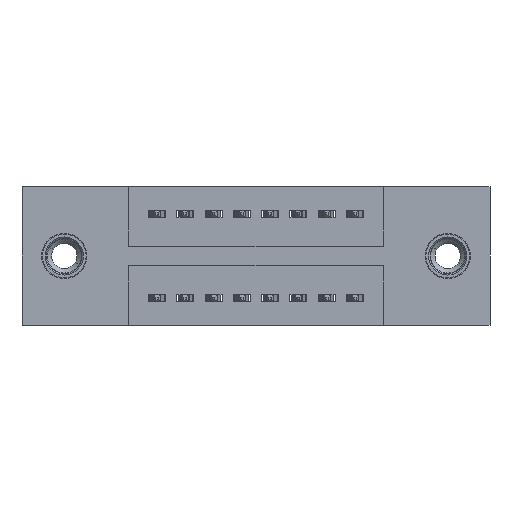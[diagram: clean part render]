
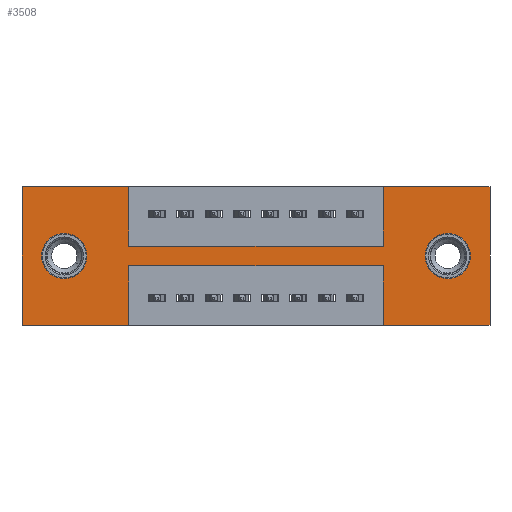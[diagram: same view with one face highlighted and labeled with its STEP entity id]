
A CAD part, front view. The second image highlights one B-rep face of the part: STEP entity #3508.
In plain terms, the highlighted planar face has unit normal (0, -1, 0).
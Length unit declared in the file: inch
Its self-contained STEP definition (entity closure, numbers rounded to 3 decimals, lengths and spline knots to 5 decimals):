
#257 = VERTEX_POINT ( 'NONE', #9334 ) ;
#258 = DIRECTION ( 'NONE',  ( 0., 1., 0. ) ) ;
#291 = CARTESIAN_POINT ( 'NONE',  ( 0.3775, 0., -0.28 ) ) ;
#521 = EDGE_CURVE ( 'NONE', #3540, #8473, #681, .T. ) ;
#585 = CARTESIAN_POINT ( 'NONE',  ( 1.655, 0., 0. ) ) ;
#623 = CARTESIAN_POINT ( 'NONE',  ( 1.655, 0., 0. ) ) ;
#681 = LINE ( 'NONE', #2844, #2631 ) ;
#764 = AXIS2_PLACEMENT_3D ( 'NONE', #10025, #2555, #10059 ) ;
#872 = EDGE_LOOP ( 'NONE', ( #3170, #6755 ) ) ;
#934 = DIRECTION ( 'NONE',  ( -1., 0., 0. ) ) ;
#1196 = ORIENTED_EDGE ( 'NONE', *, *, #9665, .F. ) ;
#1228 = CARTESIAN_POINT ( 'NONE',  ( 0., 0., -0.49 ) ) ;
#1275 = LINE ( 'NONE', #1695, #3624 ) ;
#1340 = VECTOR ( 'NONE', #8317, 39.37008 ) ;
#1508 = VERTEX_POINT ( 'NONE', #7188 ) ;
#1526 = LINE ( 'NONE', #4250, #10143 ) ;
#1599 = VERTEX_POINT ( 'NONE', #10474 ) ;
#1629 = VERTEX_POINT ( 'NONE', #10762 ) ;
#1646 = EDGE_CURVE ( 'NONE', #1508, #257, #7948, .T. ) ;
#1695 = CARTESIAN_POINT ( 'NONE',  ( 0., 0., -0.49 ) ) ;
#1846 = VECTOR ( 'NONE', #7177, 39.37008 ) ;
#1883 = DIRECTION ( 'NONE',  ( 0., 1., 0. ) ) ;
#2124 = CARTESIAN_POINT ( 'NONE',  ( 0., 0., 0. ) ) ;
#2167 = DIRECTION ( 'NONE',  ( 0., 0., -1. ) ) ;
#2207 = EDGE_CURVE ( 'NONE', #7384, #5151, #1275, .T. ) ;
#2238 = ORIENTED_EDGE ( 'NONE', *, *, #1646, .T. ) ;
#2365 = DIRECTION ( 'NONE',  ( 0., 0., -1. ) ) ;
#2447 = CIRCLE ( 'NONE', #764, 0.08 ) ;
#2555 = DIRECTION ( 'NONE',  ( 0., 1., 0. ) ) ;
#2631 = VECTOR ( 'NONE', #10314, 39.37008 ) ;
#2638 = CARTESIAN_POINT ( 'NONE',  ( 1.5055, 0., -0.245 ) ) ;
#2647 = ORIENTED_EDGE ( 'NONE', *, *, #8087, .F. ) ;
#2670 = ORIENTED_EDGE ( 'NONE', *, *, #3336, .F. ) ;
#2773 = EDGE_CURVE ( 'NONE', #7735, #1629, #1526, .T. ) ;
#2844 = CARTESIAN_POINT ( 'NONE',  ( 0., 0., -0.49 ) ) ;
#3000 = VERTEX_POINT ( 'NONE', #10274 ) ;
#3110 = AXIS2_PLACEMENT_3D ( 'NONE', #6658, #6697, #7510 ) ;
#3155 = CIRCLE ( 'NONE', #3383, 0.08 ) ;
#3166 = EDGE_LOOP ( 'NONE', ( #4093, #2238 ) ) ;
#3170 = ORIENTED_EDGE ( 'NONE', *, *, #5149, .T. ) ;
#3336 = EDGE_CURVE ( 'NONE', #1599, #9277, #3474, .T. ) ;
#3383 = AXIS2_PLACEMENT_3D ( 'NONE', #8575, #1883, #10221 ) ;
#3471 = VECTOR ( 'NONE', #2167, 39.37008 ) ;
#3474 = LINE ( 'NONE', #6778, #10266 ) ;
#3477 = ORIENTED_EDGE ( 'NONE', *, *, #2773, .F. ) ;
#3508 = ADVANCED_FACE ( 'NONE', ( #10252, #8301, #4794 ), #3770, .T. ) ;
#3540 = VERTEX_POINT ( 'NONE', #10417 ) ;
#3578 = CIRCLE ( 'NONE', #3110, 0.08 ) ;
#3624 = VECTOR ( 'NONE', #934, 39.37008 ) ;
#3767 = ORIENTED_EDGE ( 'NONE', *, *, #7443, .F. ) ;
#3770 = PLANE ( 'NONE',  #7079 ) ;
#3809 = DIRECTION ( 'NONE',  ( 0., 0., -1. ) ) ;
#3821 = LINE ( 'NONE', #4916, #1340 ) ;
#3827 = ORIENTED_EDGE ( 'NONE', *, *, #2207, .F. ) ;
#3902 = VECTOR ( 'NONE', #9910, 39.37008 ) ;
#4040 = CARTESIAN_POINT ( 'NONE',  ( 0.1495, 0., -0.325 ) ) ;
#4093 = ORIENTED_EDGE ( 'NONE', *, *, #6810, .T. ) ;
#4250 = CARTESIAN_POINT ( 'NONE',  ( 0.3775, 0., -0.21 ) ) ;
#4261 = VERTEX_POINT ( 'NONE', #2124 ) ;
#4711 = VECTOR ( 'NONE', #7700, 39.37008 ) ;
#4794 = FACE_OUTER_BOUND ( 'NONE', #6823, .T. ) ;
#4851 = CARTESIAN_POINT ( 'NONE',  ( 0.3775, 0., -0.21 ) ) ;
#4916 = CARTESIAN_POINT ( 'NONE',  ( 1.2775, 0., -0.28 ) ) ;
#5149 = EDGE_CURVE ( 'NONE', #8597, #8641, #3578, .T. ) ;
#5151 = VERTEX_POINT ( 'NONE', #5787 ) ;
#5195 = DIRECTION ( 'NONE',  ( 1., 0., 0. ) ) ;
#5590 = AXIS2_PLACEMENT_3D ( 'NONE', #2638, #258, #7625 ) ;
#5622 = CARTESIAN_POINT ( 'NONE',  ( 1.2775, 0., -0.28 ) ) ;
#5635 = CARTESIAN_POINT ( 'NONE',  ( 0.1495, 0., -0.165 ) ) ;
#5787 = CARTESIAN_POINT ( 'NONE',  ( 0., 0., -0.49 ) ) ;
#6047 = ORIENTED_EDGE ( 'NONE', *, *, #8840, .F. ) ;
#6208 = CARTESIAN_POINT ( 'NONE',  ( 0.3775, 0., -0.21 ) ) ;
#6264 = DIRECTION ( 'NONE',  ( 0., 0., 1. ) ) ;
#6373 = CARTESIAN_POINT ( 'NONE',  ( 1.2775, 0., -0.49 ) ) ;
#6527 = VECTOR ( 'NONE', #6264, 39.37008 ) ;
#6539 = CARTESIAN_POINT ( 'NONE',  ( 0.3775, 0., -0.28 ) ) ;
#6564 = VECTOR ( 'NONE', #8232, 39.37008 ) ;
#6658 = CARTESIAN_POINT ( 'NONE',  ( 0.1495, 0., -0.245 ) ) ;
#6697 = DIRECTION ( 'NONE',  ( 0., 1., 0. ) ) ;
#6714 = LINE ( 'NONE', #4851, #9725 ) ;
#6755 = ORIENTED_EDGE ( 'NONE', *, *, #9466, .T. ) ;
#6778 = CARTESIAN_POINT ( 'NONE',  ( 0., 0., 0. ) ) ;
#6810 = EDGE_CURVE ( 'NONE', #257, #1508, #2447, .T. ) ;
#6823 = EDGE_LOOP ( 'NONE', ( #8211, #3477, #3767, #6047, #1196, #3827, #7851, #9543, #2647, #9557, #7418, #2670 ) ) ;
#7079 = AXIS2_PLACEMENT_3D ( 'NONE', #1228, #10451, #3809 ) ;
#7145 = EDGE_CURVE ( 'NONE', #9277, #3540, #7262, .T. ) ;
#7177 = DIRECTION ( 'NONE',  ( 0., 0., 1. ) ) ;
#7188 = CARTESIAN_POINT ( 'NONE',  ( 1.5055, 0., -0.325 ) ) ;
#7262 = LINE ( 'NONE', #585, #3471 ) ;
#7314 = CARTESIAN_POINT ( 'NONE',  ( 0.3775, 0., -0.49 ) ) ;
#7384 = VERTEX_POINT ( 'NONE', #7314 ) ;
#7418 = ORIENTED_EDGE ( 'NONE', *, *, #7145, .F. ) ;
#7443 = EDGE_CURVE ( 'NONE', #3000, #7735, #6714, .T. ) ;
#7510 = DIRECTION ( 'NONE',  ( 0., 0., 1. ) ) ;
#7625 = DIRECTION ( 'NONE',  ( 0., 0., -1. ) ) ;
#7700 = DIRECTION ( 'NONE',  ( -1., 0., 0. ) ) ;
#7735 = VERTEX_POINT ( 'NONE', #6208 ) ;
#7851 = ORIENTED_EDGE ( 'NONE', *, *, #10167, .F. ) ;
#7948 = CIRCLE ( 'NONE', #5590, 0.08 ) ;
#7976 = VERTEX_POINT ( 'NONE', #8904 ) ;
#8020 = CARTESIAN_POINT ( 'NONE',  ( 1.2775, 0., -0.21 ) ) ;
#8087 = EDGE_CURVE ( 'NONE', #8473, #9228, #3821, .T. ) ;
#8211 = ORIENTED_EDGE ( 'NONE', *, *, #9800, .F. ) ;
#8232 = DIRECTION ( 'NONE',  ( 1., 0., 0. ) ) ;
#8259 = LINE ( 'NONE', #9372, #6564 ) ;
#8301 = FACE_BOUND ( 'NONE', #872, .T. ) ;
#8317 = DIRECTION ( 'NONE',  ( 0., 0., 1. ) ) ;
#8471 = LINE ( 'NONE', #291, #4711 ) ;
#8473 = VERTEX_POINT ( 'NONE', #6373 ) ;
#8575 = CARTESIAN_POINT ( 'NONE',  ( 0.1495, 0., -0.245 ) ) ;
#8597 = VERTEX_POINT ( 'NONE', #5635 ) ;
#8641 = VERTEX_POINT ( 'NONE', #4040 ) ;
#8840 = EDGE_CURVE ( 'NONE', #4261, #3000, #8259, .T. ) ;
#8904 = CARTESIAN_POINT ( 'NONE',  ( 0.3775, 0., -0.28 ) ) ;
#9012 = LINE ( 'NONE', #8020, #6527 ) ;
#9228 = VERTEX_POINT ( 'NONE', #5622 ) ;
#9277 = VERTEX_POINT ( 'NONE', #623 ) ;
#9278 = DIRECTION ( 'NONE',  ( 1., 0., 0. ) ) ;
#9334 = CARTESIAN_POINT ( 'NONE',  ( 1.5055, 0., -0.165 ) ) ;
#9372 = CARTESIAN_POINT ( 'NONE',  ( 0., 0., 0. ) ) ;
#9466 = EDGE_CURVE ( 'NONE', #8641, #8597, #3155, .T. ) ;
#9543 = ORIENTED_EDGE ( 'NONE', *, *, #10445, .F. ) ;
#9557 = ORIENTED_EDGE ( 'NONE', *, *, #521, .F. ) ;
#9629 = CARTESIAN_POINT ( 'NONE',  ( 0., 0., 0. ) ) ;
#9657 = LINE ( 'NONE', #6539, #3902 ) ;
#9665 = EDGE_CURVE ( 'NONE', #5151, #4261, #9816, .T. ) ;
#9725 = VECTOR ( 'NONE', #2365, 39.37008 ) ;
#9800 = EDGE_CURVE ( 'NONE', #1629, #1599, #9012, .T. ) ;
#9816 = LINE ( 'NONE', #9629, #1846 ) ;
#9910 = DIRECTION ( 'NONE',  ( 0., 0., -1. ) ) ;
#10025 = CARTESIAN_POINT ( 'NONE',  ( 1.5055, 0., -0.245 ) ) ;
#10059 = DIRECTION ( 'NONE',  ( 0., 0., -1. ) ) ;
#10143 = VECTOR ( 'NONE', #9278, 39.37008 ) ;
#10167 = EDGE_CURVE ( 'NONE', #7976, #7384, #9657, .T. ) ;
#10221 = DIRECTION ( 'NONE',  ( 0., 0., 1. ) ) ;
#10252 = FACE_BOUND ( 'NONE', #3166, .T. ) ;
#10266 = VECTOR ( 'NONE', #5195, 39.37008 ) ;
#10274 = CARTESIAN_POINT ( 'NONE',  ( 0.3775, 0., 0. ) ) ;
#10314 = DIRECTION ( 'NONE',  ( -1., 0., 0. ) ) ;
#10417 = CARTESIAN_POINT ( 'NONE',  ( 1.655, 0., -0.49 ) ) ;
#10445 = EDGE_CURVE ( 'NONE', #9228, #7976, #8471, .T. ) ;
#10451 = DIRECTION ( 'NONE',  ( 0., -1., 0. ) ) ;
#10474 = CARTESIAN_POINT ( 'NONE',  ( 1.2775, 0., 0. ) ) ;
#10762 = CARTESIAN_POINT ( 'NONE',  ( 1.2775, 0., -0.21 ) ) ;
